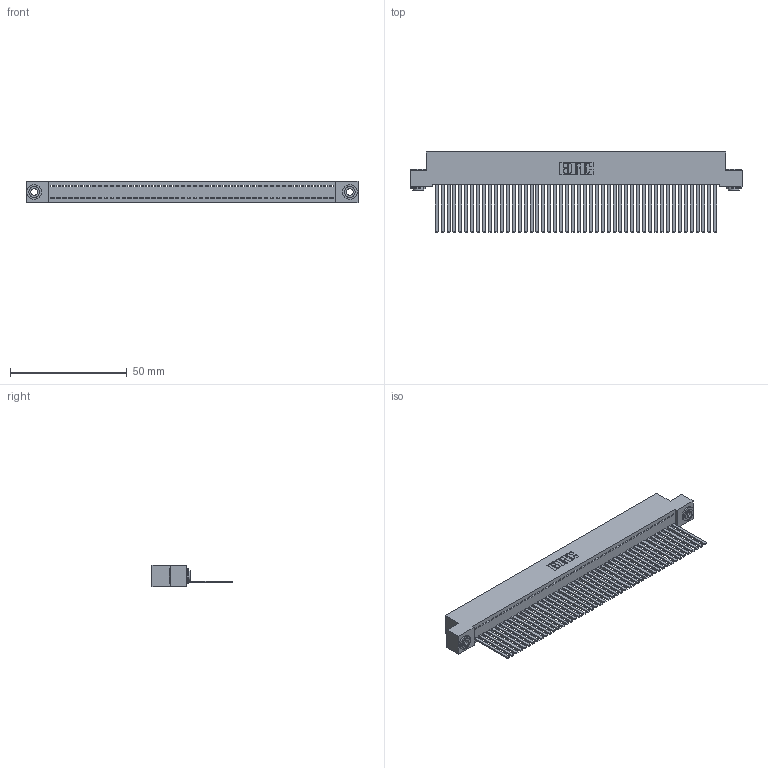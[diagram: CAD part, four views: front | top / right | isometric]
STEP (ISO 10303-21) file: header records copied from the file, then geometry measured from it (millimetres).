
FILE_DESCRIPTION (( 'STEP AP203' ), '1' );
FILE_NAME ('342-048-544-103.STEP', '2018-08-12T18:11:50', ( '' ), ( '' ), 'SwSTEP 2.0', 'SolidWorks 2016', '' );
FILE_SCHEMA (( 'CONFIG_CONTROL_DESIGN' ));
Length unit declared in the file: inch
Products named in the file (4): 342 Part_.156 TH; 345-292-001_345-293-144; 342-250-002_345-250-002-102; 342-048-544-103
Assembly tree (51 placements, depth 2):
  342-048-544-103
    342 Part_.156 TH
    345-292-001_345-293-144  x48
    342-250-002_345-250-002-102  x2
Bounding box: 142.24 x 34.3 x 9.4 mm (x, y, z)
Volume: 13072.4 mm3; surface area: 21116.6 mm2
Topology: 51 solids, 51 shells, 2644 faces, 7959 edges, 5238 vertices
Faces by surface type: plane 1900, cylinder 736, cone 8
Entity records: 28902 total; most frequent: CARTESIAN_POINT 4961, ORIENTED_EDGE 4938, DIRECTION 4203, EDGE_CURVE 2469, VECTOR 2321, LINE 2321, VERTEX_POINT 1642, AXIS2_PLACEMENT_3D 941
